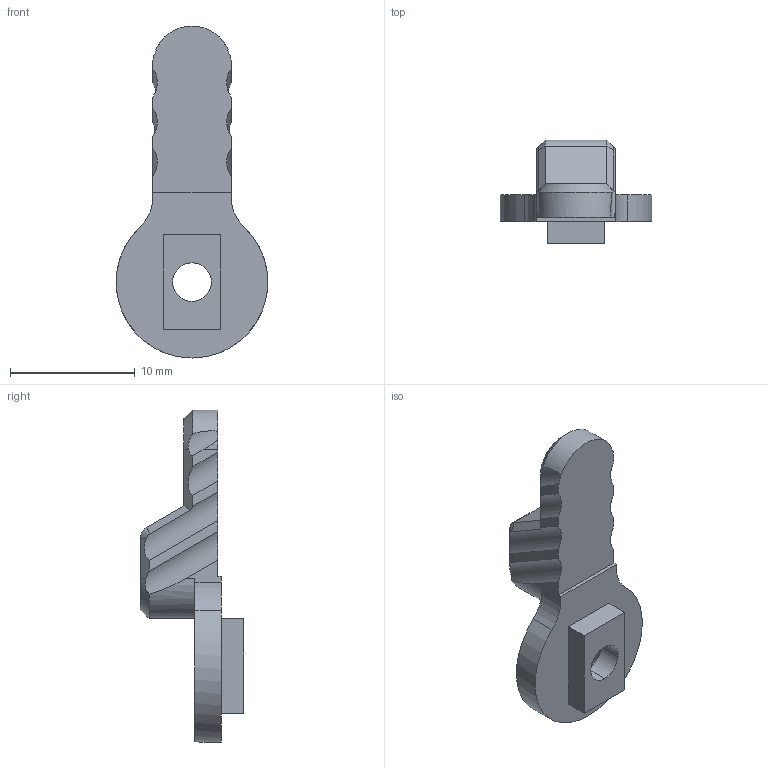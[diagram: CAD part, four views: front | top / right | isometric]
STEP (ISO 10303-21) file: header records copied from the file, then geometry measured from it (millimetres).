
FILE_DESCRIPTION (( 'STEP AP214' ), '1' );
FILE_NAME ('Lever_Hybrid.step', '2015-07-11T17:33:16', ( 'WarFairy' ), ( '' ), 'SwSTEP 2.0', 'SolidWorks 2015', '' );
FILE_SCHEMA (( 'AUTOMOTIVE_DESIGN' ));
Length unit declared in the file: millimetre
Products named in the file (1): Lever_Hybrid
Bounding box: 12.17 x 8.29 x 26.63 mm (x, y, z)
Volume: 635.8 mm3; surface area: 707.4 mm2
Topology: 1 solids, 1 shells, 67 faces, 180 edges, 114 vertices
Faces by surface type: plane 31, cylinder 22, cone 10, torus 4
Entity records: 2149 total; most frequent: CARTESIAN_POINT 501, ORIENTED_EDGE 354, DIRECTION 323, EDGE_CURVE 177, VERTEX_POINT 114, AXIS2_PLACEMENT_3D 112, LINE 99, VECTOR 99
